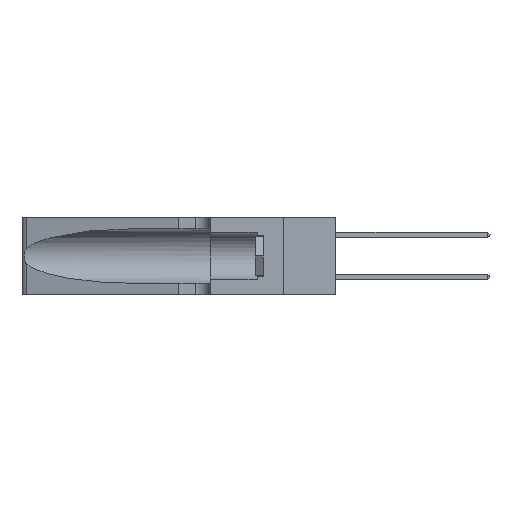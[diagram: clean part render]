
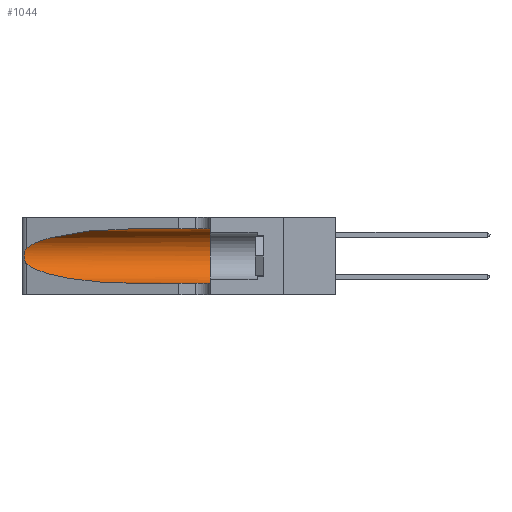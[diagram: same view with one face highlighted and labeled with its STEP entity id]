
A CAD part, left-side view. The second image highlights one B-rep face of the part: STEP entity #1044.
In plain terms, the highlighted cylindrical face has radius 3.308 mm (diameter 6.617 mm), a partial arc.
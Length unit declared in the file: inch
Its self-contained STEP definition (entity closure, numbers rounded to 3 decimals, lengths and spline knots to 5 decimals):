
#734 = CARTESIAN_POINT ( 'NONE',  ( 0.25487, 1.22718, 0.22369 ) ) ;
#1044 = ADVANCED_FACE ( 'NONE', ( #7645 ), #39050, .F. ) ;
#1099 = CARTESIAN_POINT ( 'NONE',  ( 0.1305, 0.72297, 0.05475 ) ) ;
#1158 = VERTEX_POINT ( 'NONE', #35737 ) ;
#2041 = DIRECTION ( 'NONE',  ( 0., 0., 1. ) ) ;
#2964 = CARTESIAN_POINT ( 'NONE',  ( 0.1305, 1.61858, 0.31525 ) ) ;
#7071 = CARTESIAN_POINT ( 'NONE',  ( 0.26018, 1.23835, 0.19895 ) ) ;
#7233 = CARTESIAN_POINT ( 'NONE',  ( 0.26075, 1.23896, 0.178 ) ) ;
#7295 = CARTESIAN_POINT ( 'NONE',  ( 0.1305, 0.35, 0.05475 ) ) ;
#7516 = VERTEX_POINT ( 'NONE', #1099 ) ;
#7645 = FACE_OUTER_BOUND ( 'NONE', #34969, .T. ) ;
#9161 = EDGE_CURVE ( 'NONE', #39561, #42795, #24230, .T. ) ;
#9474 = ORIENTED_EDGE ( 'NONE', *, *, #44401, .T. ) ;
#10885 = CARTESIAN_POINT ( 'NONE',  ( 0.25555, 1.22993, 0.14849 ) ) ;
#11817 = CARTESIAN_POINT ( 'NONE',  ( 0.18966, 0.96281, 0.31525 ) ) ;
#11973 = CARTESIAN_POINT ( 'NONE',  ( 0.25487, 1.22718, 0.22369 ) ) ;
#12670 = CARTESIAN_POINT ( 'NONE',  ( 0.1305, 1.61858, 0.185 ) ) ;
#14916 = VECTOR ( 'NONE', #25131, 39.37008 ) ;
#15247 = CARTESIAN_POINT ( 'NONE',  ( 0.1305, 0.72297, 0.31525 ) ) ;
#15407 = ORIENTED_EDGE ( 'NONE', *, *, #9161, .T. ) ;
#15778 =( BOUNDED_CURVE ( )  B_SPLINE_CURVE ( 3, ( #23017, #26341, #30164, #30487 ),
 .UNSPECIFIED., .F., .T. ) 
 B_SPLINE_CURVE_WITH_KNOTS ( ( 4, 4 ),
 ( 3.44316, 4.71239 ),
 .UNSPECIFIED. ) 
 CURVE ( )  GEOMETRIC_REPRESENTATION_ITEM ( )  RATIONAL_B_SPLINE_CURVE ( ( 1., 0.87, 0.87, 1. ) ) 
 REPRESENTATION_ITEM ( '' )  );
#16784 = DIRECTION ( 'NONE',  ( 0., 0., -1. ) ) ;
#17718 = CARTESIAN_POINT ( 'NONE',  ( 0.25639, 1.23186, 0.15144 ) ) ;
#18207 = CARTESIAN_POINT ( 'NONE',  ( 0.25854, 1.2359, 0.20912 ) ) ;
#18970 = CARTESIAN_POINT ( 'NONE',  ( 0.2373, 1.15595, 0.28018 ) ) ;
#19685 = VERTEX_POINT ( 'NONE', #15247 ) ;
#20550 = ORIENTED_EDGE ( 'NONE', *, *, #39234, .F. ) ;
#21546 = CARTESIAN_POINT ( 'NONE',  ( 0.25639, 1.23184, 0.21858 ) ) ;
#22314 = LINE ( 'NONE', #2964, #14916 ) ;
#23017 = CARTESIAN_POINT ( 'NONE',  ( 0.25487, 1.22718, 0.14631 ) ) ;
#24230 = B_SPLINE_CURVE_WITH_KNOTS ( 'NONE', 3,
 ( #32381, #39945, #21546, #46677, #18207, #7071, #32540, #7233, #39621, #43628, #29042, #17718, #10885, #36410 ),
 .UNSPECIFIED., .F., .F.,
 ( 4, 2, 2, 2, 2, 2, 4 ),
 ( 0., 0.00027, 0.00053, 0.00107, 0.0016, 0.00187, 0.00214 ),
 .UNSPECIFIED. ) ;
#24770 = EDGE_CURVE ( 'NONE', #7516, #39483, #30233, .T. ) ;
#25131 = DIRECTION ( 'NONE',  ( 0., -1., 0. ) ) ;
#25214 = ORIENTED_EDGE ( 'NONE', *, *, #24770, .T. ) ;
#26341 = CARTESIAN_POINT ( 'NONE',  ( 0.2373, 1.15595, 0.08982 ) ) ;
#26809 = AXIS2_PLACEMENT_3D ( 'NONE', #12670, #41898, #16784 ) ;
#29042 = CARTESIAN_POINT ( 'NONE',  ( 0.25789, 1.23486, 0.15765 ) ) ;
#30164 = CARTESIAN_POINT ( 'NONE',  ( 0.18966, 0.96281, 0.05475 ) ) ;
#30233 = LINE ( 'NONE', #34120, #38842 ) ;
#30487 = CARTESIAN_POINT ( 'NONE',  ( 0.1305, 0.72297, 0.05475 ) ) ;
#30891 = ORIENTED_EDGE ( 'NONE', *, *, #46785, .F. ) ;
#32381 = CARTESIAN_POINT ( 'NONE',  ( 0.25487, 1.22718, 0.22369 ) ) ;
#32540 = CARTESIAN_POINT ( 'NONE',  ( 0.26075, 1.23896, 0.19203 ) ) ;
#34120 = CARTESIAN_POINT ( 'NONE',  ( 0.1305, 1.61858, 0.05475 ) ) ;
#34235 = CARTESIAN_POINT ( 'NONE',  ( 0.25487, 1.22718, 0.14631 ) ) ;
#34969 = EDGE_LOOP ( 'NONE', ( #9474, #15407, #39326, #25214, #30891, #20550 ) ) ;
#35178 = CIRCLE ( 'NONE', #46844, 0.13025 ) ;
#35737 = CARTESIAN_POINT ( 'NONE',  ( 0.1305, 0.35, 0.31525 ) ) ;
#36410 = CARTESIAN_POINT ( 'NONE',  ( 0.25487, 1.22718, 0.14631 ) ) ;
#38842 = VECTOR ( 'NONE', #41048, 39.37008 ) ;
#39050 = CYLINDRICAL_SURFACE ( 'NONE', #26809, 0.13025 ) ;
#39234 = EDGE_CURVE ( 'NONE', #19685, #1158, #22314, .T. ) ;
#39326 = ORIENTED_EDGE ( 'NONE', *, *, #45939, .T. ) ;
#39483 = VERTEX_POINT ( 'NONE', #7295 ) ;
#39561 = VERTEX_POINT ( 'NONE', #734 ) ;
#39621 = CARTESIAN_POINT ( 'NONE',  ( 0.26017, 1.23833, 0.17102 ) ) ;
#39945 = CARTESIAN_POINT ( 'NONE',  ( 0.25555, 1.22994, 0.2215 ) ) ;
#41048 = DIRECTION ( 'NONE',  ( 0., -1., 0. ) ) ;
#41898 = DIRECTION ( 'NONE',  ( 0., -1., 0. ) ) ;
#41987 = CARTESIAN_POINT ( 'NONE',  ( 0.1305, 0.35, 0.185 ) ) ;
#42795 = VERTEX_POINT ( 'NONE', #34235 ) ;
#43439 = CARTESIAN_POINT ( 'NONE',  ( 0.1305, 0.72297, 0.31525 ) ) ;
#43628 = CARTESIAN_POINT ( 'NONE',  ( 0.25856, 1.23593, 0.16098 ) ) ;
#44401 = EDGE_CURVE ( 'NONE', #19685, #39561, #44749, .T. ) ;
#44749 =( BOUNDED_CURVE ( )  B_SPLINE_CURVE ( 3, ( #43439, #11817, #18970, #11973 ),
 .UNSPECIFIED., .F., .F. ) 
 B_SPLINE_CURVE_WITH_KNOTS ( ( 4, 4 ),
 ( 1.5708, 2.84003 ),
 .UNSPECIFIED. ) 
 CURVE ( )  GEOMETRIC_REPRESENTATION_ITEM ( )  RATIONAL_B_SPLINE_CURVE ( ( 1., 0.87, 0.87, 1. ) ) 
 REPRESENTATION_ITEM ( '' )  );
#45939 = EDGE_CURVE ( 'NONE', #42795, #7516, #15778, .T. ) ;
#46117 = DIRECTION ( 'NONE',  ( 0., 1., 0. ) ) ;
#46677 = CARTESIAN_POINT ( 'NONE',  ( 0.25787, 1.23484, 0.2124 ) ) ;
#46785 = EDGE_CURVE ( 'NONE', #1158, #39483, #35178, .T. ) ;
#46844 = AXIS2_PLACEMENT_3D ( 'NONE', #41987, #46117, #2041 ) ;
